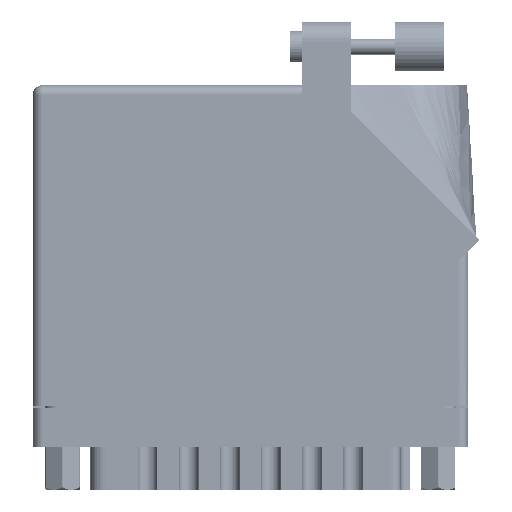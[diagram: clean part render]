
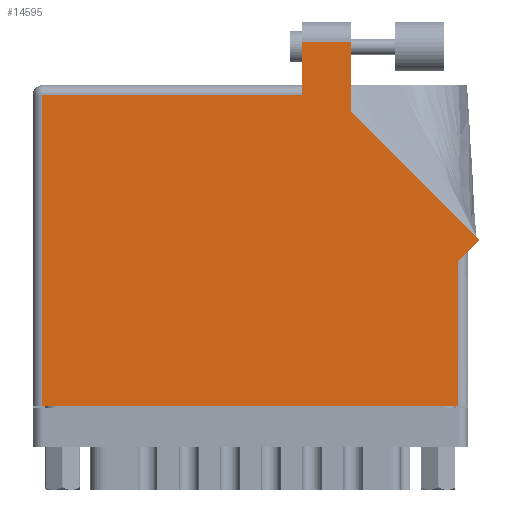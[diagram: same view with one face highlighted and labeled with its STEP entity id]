
A CAD part, front view. The second image highlights one B-rep face of the part: STEP entity #14595.
In plain terms, the highlighted face is planar.
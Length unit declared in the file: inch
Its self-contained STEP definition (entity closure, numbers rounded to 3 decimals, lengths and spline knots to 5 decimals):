
#1492 = VERTEX_POINT ( 'NONE', #54723 ) ;
#5674 = CARTESIAN_POINT ( 'NONE',  ( 1.705, 1.968, 0. ) ) ;
#7476 = DIRECTION ( 'NONE',  ( 0.707, 0.707, 0. ) ) ;
#7607 = ORIENTED_EDGE ( 'NONE', *, *, #22947, .T. ) ;
#8097 = LINE ( 'NONE', #100071, #104192 ) ;
#9115 = VERTEX_POINT ( 'NONE', #39538 ) ;
#11436 = DIRECTION ( 'NONE',  ( -1., 0., 0. ) ) ;
#11987 = ORIENTED_EDGE ( 'NONE', *, *, #70330, .T. ) ;
#11988 = CARTESIAN_POINT ( 'NONE',  ( 2.693, 0.918, 0. ) ) ;
#13554 = VERTEX_POINT ( 'NONE', #79982 ) ;
#13997 = DIRECTION ( 'NONE',  ( -1., 0., 0. ) ) ;
#14290 = DIRECTION ( 'NONE',  ( 0., -1., 0. ) ) ;
#14595 = ADVANCED_FACE ( 'NONE', ( #103819 ), #103914, .F. ) ;
#17520 = LINE ( 'NONE', #93886, #81643 ) ;
#18186 = CARTESIAN_POINT ( 'NONE',  ( 2.755, 0.98, 0. ) ) ;
#18603 = LINE ( 'NONE', #105515, #60975 ) ;
#18753 = LINE ( 'NONE', #100370, #45686 ) ;
#19149 = VERTEX_POINT ( 'NONE', #20805 ) ;
#20805 = CARTESIAN_POINT ( 'NONE',  ( 2.012, 1.86442, 0. ) ) ;
#21587 = VERTEX_POINT ( 'NONE', #5674 ) ;
#22045 = VECTOR ( 'NONE', #104447, 39.37008 ) ;
#22947 = EDGE_CURVE ( 'NONE', #66149, #62848, #32228, .T. ) ;
#24230 = DIRECTION ( 'NONE',  ( -1., 0., 0. ) ) ;
#25993 = ORIENTED_EDGE ( 'NONE', *, *, #38739, .T. ) ;
#26220 = DIRECTION ( 'NONE',  ( -0.707, 0.707, 0. ) ) ;
#27085 = EDGE_CURVE ( 'NONE', #1492, #35869, #55679, .T. ) ;
#30193 = CARTESIAN_POINT ( 'NONE',  ( 2.82571, 1.05071, 0. ) ) ;
#31800 = EDGE_CURVE ( 'NONE', #62848, #19149, #18753, .T. ) ;
#32058 = CARTESIAN_POINT ( 'NONE',  ( 2.012, 1.86442, 0. ) ) ;
#32092 = CARTESIAN_POINT ( 'NONE',  ( 1.705, 2.03, 0. ) ) ;
#32228 = LINE ( 'NONE', #18186, #86110 ) ;
#33624 = ORIENTED_EDGE ( 'NONE', *, *, #46811, .T. ) ;
#35159 = ORIENTED_EDGE ( 'NONE', *, *, #31800, .T. ) ;
#35869 = VERTEX_POINT ( 'NONE', #43714 ) ;
#38739 = EDGE_CURVE ( 'NONE', #94007, #66149, #18603, .T. ) ;
#39367 = AXIS2_PLACEMENT_3D ( 'NONE', #54838, #53806, #13997 ) ;
#39538 = CARTESIAN_POINT ( 'NONE',  ( 1.705, 2.305, 0. ) ) ;
#39929 = DIRECTION ( 'NONE',  ( 0., 1., 0. ) ) ;
#43714 = CARTESIAN_POINT ( 'NONE',  ( 0.062, 0., 0. ) ) ;
#45588 = LINE ( 'NONE', #80916, #103257 ) ;
#45686 = VECTOR ( 'NONE', #26220, 39.37008 ) ;
#46811 = EDGE_CURVE ( 'NONE', #19149, #13554, #60007, .T. ) ;
#53806 = DIRECTION ( 'NONE',  ( 0., 0., -1. ) ) ;
#54723 = CARTESIAN_POINT ( 'NONE',  ( 0.062, 1.968, 0. ) ) ;
#54838 = CARTESIAN_POINT ( 'NONE',  ( 0., 2.03, 0. ) ) ;
#55679 = LINE ( 'NONE', #71271, #76191 ) ;
#56452 = DIRECTION ( 'NONE',  ( 0., 1., 0. ) ) ;
#56763 = ORIENTED_EDGE ( 'NONE', *, *, #27085, .T. ) ;
#60007 = LINE ( 'NONE', #32058, #84429 ) ;
#60975 = VECTOR ( 'NONE', #56452, 39.37008 ) ;
#62848 = VERTEX_POINT ( 'NONE', #30193 ) ;
#66149 = VERTEX_POINT ( 'NONE', #11988 ) ;
#68217 = DIRECTION ( 'NONE',  ( 1., 0., 0. ) ) ;
#70330 = EDGE_CURVE ( 'NONE', #13554, #9115, #45588, .T. ) ;
#71271 = CARTESIAN_POINT ( 'NONE',  ( 0.062, 0., 0. ) ) ;
#72441 = CARTESIAN_POINT ( 'NONE',  ( 2.693, 0., 0. ) ) ;
#73422 = EDGE_CURVE ( 'NONE', #21587, #1492, #17520, .T. ) ;
#74131 = ORIENTED_EDGE ( 'NONE', *, *, #73422, .T. ) ;
#75540 = EDGE_CURVE ( 'NONE', #35869, #94007, #8097, .T. ) ;
#76191 = VECTOR ( 'NONE', #14290, 39.37008 ) ;
#79982 = CARTESIAN_POINT ( 'NONE',  ( 2.012, 2.305, 0. ) ) ;
#80916 = CARTESIAN_POINT ( 'NONE',  ( 1.705, 2.305, 0. ) ) ;
#81106 = LINE ( 'NONE', #32092, #22045 ) ;
#81635 = EDGE_LOOP ( 'NONE', ( #33624, #11987, #105036, #74131, #56763, #88117, #25993, #7607, #35159 ) ) ;
#81643 = VECTOR ( 'NONE', #11436, 39.37008 ) ;
#82570 = EDGE_CURVE ( 'NONE', #9115, #21587, #81106, .T. ) ;
#84429 = VECTOR ( 'NONE', #39929, 39.37008 ) ;
#86110 = VECTOR ( 'NONE', #7476, 39.37008 ) ;
#88117 = ORIENTED_EDGE ( 'NONE', *, *, #75540, .T. ) ;
#93886 = CARTESIAN_POINT ( 'NONE',  ( 0., 1.968, 0. ) ) ;
#94007 = VERTEX_POINT ( 'NONE', #72441 ) ;
#100071 = CARTESIAN_POINT ( 'NONE',  ( 0., 0., 0. ) ) ;
#100370 = CARTESIAN_POINT ( 'NONE',  ( 2.82571, 1.05071, 0. ) ) ;
#103257 = VECTOR ( 'NONE', #24230, 39.37008 ) ;
#103819 = FACE_OUTER_BOUND ( 'NONE', #81635, .T. ) ;
#103914 = PLANE ( 'NONE',  #39367 ) ;
#104192 = VECTOR ( 'NONE', #68217, 39.37008 ) ;
#104447 = DIRECTION ( 'NONE',  ( 0., -1., 0. ) ) ;
#105036 = ORIENTED_EDGE ( 'NONE', *, *, #82570, .T. ) ;
#105515 = CARTESIAN_POINT ( 'NONE',  ( 2.693, 0.98, 0. ) ) ;
